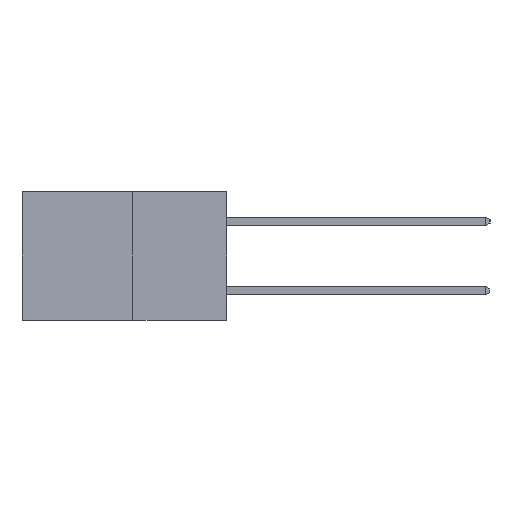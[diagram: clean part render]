
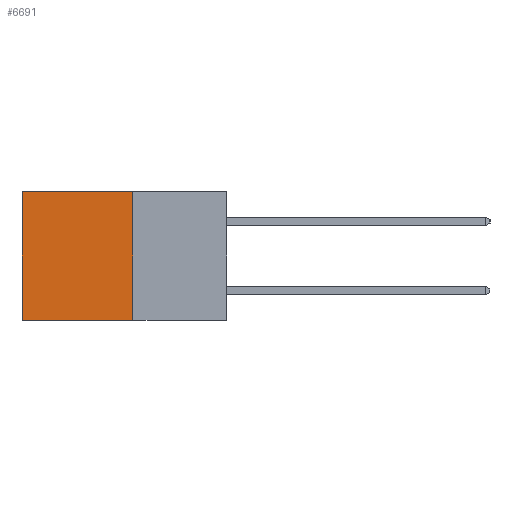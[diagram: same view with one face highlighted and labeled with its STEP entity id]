
A CAD part, left-side view. The second image highlights one B-rep face of the part: STEP entity #6691.
In plain terms, the highlighted planar face has unit normal (-1, 0, 0).
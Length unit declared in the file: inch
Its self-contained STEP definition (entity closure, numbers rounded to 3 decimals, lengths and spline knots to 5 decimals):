
#32 = DIRECTION ( 'NONE',  ( 0., 0., -1. ) ) ;
#133 = PLANE ( 'NONE',  #10757 ) ;
#479 = ORIENTED_EDGE ( 'NONE', *, *, #7191, .F. ) ;
#1349 = DIRECTION ( 'NONE',  ( 1., 0., 0. ) ) ;
#1880 = LINE ( 'NONE', #2493, #7832 ) ;
#2493 = CARTESIAN_POINT ( 'NONE',  ( 0.277, 0.27, 0. ) ) ;
#3726 = EDGE_LOOP ( 'NONE', ( #8314, #11108, #479, #12364 ) ) ;
#5451 = CARTESIAN_POINT ( 'NONE',  ( 0.277, 0.27, 0. ) ) ;
#5526 = VECTOR ( 'NONE', #32, 39.37008 ) ;
#5552 = CARTESIAN_POINT ( 'NONE',  ( 0.277, 0.59, 0. ) ) ;
#5639 = EDGE_CURVE ( 'NONE', #9350, #8383, #8177, .T. ) ;
#5867 = CARTESIAN_POINT ( 'NONE',  ( 0.277, 0.59, -0.37 ) ) ;
#6538 = DIRECTION ( 'NONE',  ( 0., 0., -1. ) ) ;
#6540 = DIRECTION ( 'NONE',  ( 0., 1., 0. ) ) ;
#6691 = ADVANCED_FACE ( 'NONE', ( #8138 ), #133, .F. ) ;
#7191 = EDGE_CURVE ( 'NONE', #10246, #9350, #7961, .T. ) ;
#7687 = CARTESIAN_POINT ( 'NONE',  ( 0.277, 0.27, -0.37 ) ) ;
#7832 = VECTOR ( 'NONE', #9848, 39.37008 ) ;
#7961 = LINE ( 'NONE', #10688, #13143 ) ;
#8035 = EDGE_CURVE ( 'NONE', #10391, #8383, #11080, .T. ) ;
#8138 = FACE_OUTER_BOUND ( 'NONE', #3726, .T. ) ;
#8177 = LINE ( 'NONE', #12732, #11279 ) ;
#8314 = ORIENTED_EDGE ( 'NONE', *, *, #8035, .T. ) ;
#8383 = VERTEX_POINT ( 'NONE', #5867 ) ;
#8766 = DIRECTION ( 'NONE',  ( 0., 0., -1. ) ) ;
#9350 = VERTEX_POINT ( 'NONE', #9636 ) ;
#9636 = CARTESIAN_POINT ( 'NONE',  ( 0.277, 0.27, -0.37 ) ) ;
#9848 = DIRECTION ( 'NONE',  ( 0., 1., 0. ) ) ;
#10246 = VERTEX_POINT ( 'NONE', #5451 ) ;
#10391 = VERTEX_POINT ( 'NONE', #5552 ) ;
#10688 = CARTESIAN_POINT ( 'NONE',  ( 0.277, 0.27, -0.37 ) ) ;
#10757 = AXIS2_PLACEMENT_3D ( 'NONE', #7687, #1349, #8766 ) ;
#11080 = LINE ( 'NONE', #12757, #5526 ) ;
#11108 = ORIENTED_EDGE ( 'NONE', *, *, #5639, .F. ) ;
#11279 = VECTOR ( 'NONE', #6540, 39.37008 ) ;
#12364 = ORIENTED_EDGE ( 'NONE', *, *, #12976, .T. ) ;
#12732 = CARTESIAN_POINT ( 'NONE',  ( 0.277, 0.27, -0.37 ) ) ;
#12757 = CARTESIAN_POINT ( 'NONE',  ( 0.277, 0.59, -0.37 ) ) ;
#12976 = EDGE_CURVE ( 'NONE', #10246, #10391, #1880, .T. ) ;
#13143 = VECTOR ( 'NONE', #6538, 39.37008 ) ;
